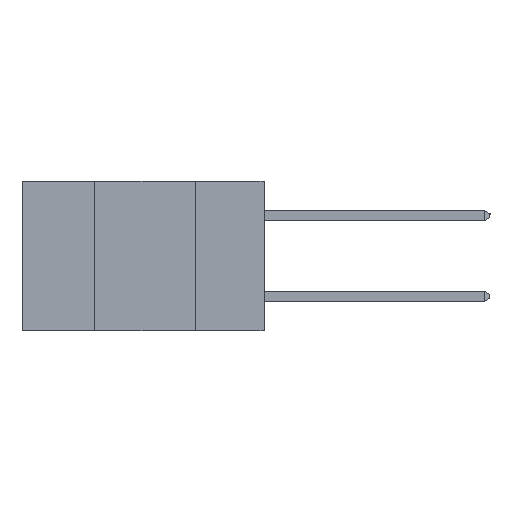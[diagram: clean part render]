
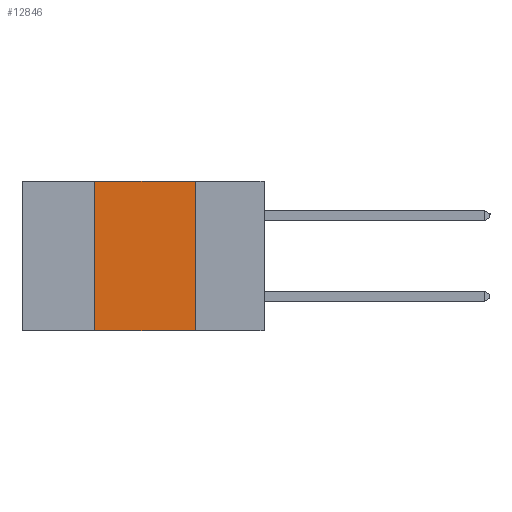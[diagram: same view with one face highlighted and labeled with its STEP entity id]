
A CAD part, left-side view. The second image highlights one B-rep face of the part: STEP entity #12846.
In plain terms, the highlighted planar face has unit normal (-1, 0, 0).
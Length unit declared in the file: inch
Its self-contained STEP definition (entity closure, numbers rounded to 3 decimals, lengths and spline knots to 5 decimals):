
#409 = LINE ( 'NONE', #8878, #5933 ) ;
#492 = VECTOR ( 'NONE', #4017, 39.37008 ) ;
#762 = FACE_OUTER_BOUND ( 'NONE', #5840, .T. ) ;
#1535 = DIRECTION ( 'NONE',  ( 0., 0., -1. ) ) ;
#1655 = ORIENTED_EDGE ( 'NONE', *, *, #8039, .T. ) ;
#1712 = VECTOR ( 'NONE', #1535, 39.37008 ) ;
#1997 = EDGE_CURVE ( 'NONE', #13145, #2456, #9019, .T. ) ;
#2456 = VERTEX_POINT ( 'NONE', #4720 ) ;
#2635 = LINE ( 'NONE', #12552, #492 ) ;
#2811 = VECTOR ( 'NONE', #4206, 39.37008 ) ;
#2938 = DIRECTION ( 'NONE',  ( 0., 0., -1. ) ) ;
#3878 = VERTEX_POINT ( 'NONE', #5077 ) ;
#4017 = DIRECTION ( 'NONE',  ( 0., -1., 0. ) ) ;
#4206 = DIRECTION ( 'NONE',  ( 0., 0., 1. ) ) ;
#4438 = ORIENTED_EDGE ( 'NONE', *, *, #1997, .F. ) ;
#4720 = CARTESIAN_POINT ( 'NONE',  ( 0., 0.17, -0.37 ) ) ;
#5005 = EDGE_CURVE ( 'NONE', #3878, #12083, #9510, .T. ) ;
#5077 = CARTESIAN_POINT ( 'NONE',  ( 0., 0.42, -0.37 ) ) ;
#5840 = EDGE_LOOP ( 'NONE', ( #4438, #9495, #11367, #1655 ) ) ;
#5933 = VECTOR ( 'NONE', #10907, 39.37008 ) ;
#6948 = AXIS2_PLACEMENT_3D ( 'NONE', #11390, #7060, #2938 ) ;
#7060 = DIRECTION ( 'NONE',  ( 1., 0., 0. ) ) ;
#8039 = EDGE_CURVE ( 'NONE', #3878, #2456, #409, .T. ) ;
#8878 = CARTESIAN_POINT ( 'NONE',  ( 0., 0.6, -0.37 ) ) ;
#9003 = CARTESIAN_POINT ( 'NONE',  ( 0., 0.17, 0. ) ) ;
#9019 = LINE ( 'NONE', #9090, #1712 ) ;
#9090 = CARTESIAN_POINT ( 'NONE',  ( 0., 0.17, -0.37 ) ) ;
#9093 = PLANE ( 'NONE',  #6948 ) ;
#9332 = CARTESIAN_POINT ( 'NONE',  ( 0., 0.42, 0. ) ) ;
#9495 = ORIENTED_EDGE ( 'NONE', *, *, #13808, .F. ) ;
#9510 = LINE ( 'NONE', #13788, #2811 ) ;
#10907 = DIRECTION ( 'NONE',  ( 0., -1., 0. ) ) ;
#11367 = ORIENTED_EDGE ( 'NONE', *, *, #5005, .F. ) ;
#11390 = CARTESIAN_POINT ( 'NONE',  ( 0., 0.6, 0. ) ) ;
#12083 = VERTEX_POINT ( 'NONE', #9332 ) ;
#12552 = CARTESIAN_POINT ( 'NONE',  ( 0., 0.6, 0. ) ) ;
#12846 = ADVANCED_FACE ( 'NONE', ( #762 ), #9093, .F. ) ;
#13145 = VERTEX_POINT ( 'NONE', #9003 ) ;
#13788 = CARTESIAN_POINT ( 'NONE',  ( 0., 0.42, -0.37 ) ) ;
#13808 = EDGE_CURVE ( 'NONE', #12083, #13145, #2635, .T. ) ;
